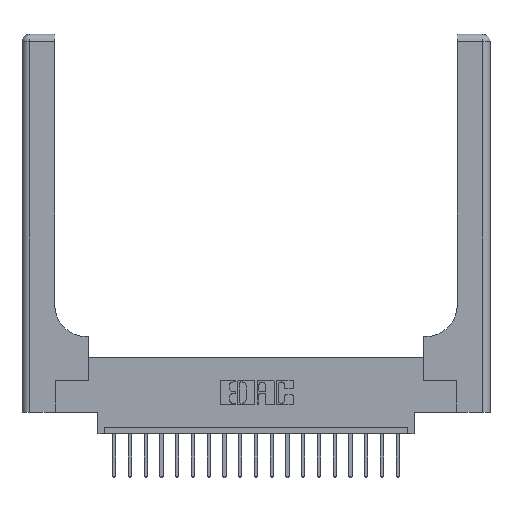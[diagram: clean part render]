
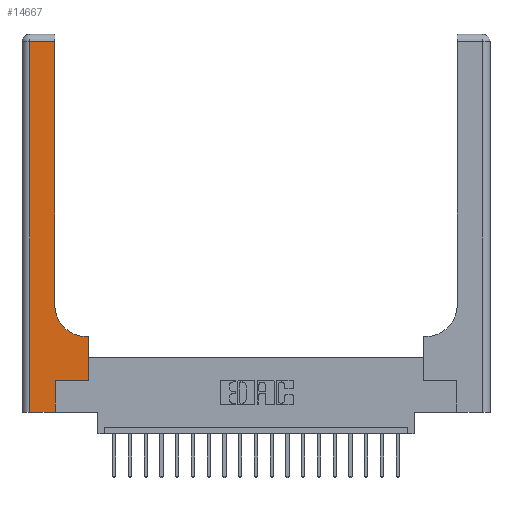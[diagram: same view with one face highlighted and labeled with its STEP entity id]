
A CAD part, top view. The second image highlights one B-rep face of the part: STEP entity #14667.
In plain terms, the highlighted planar face has unit normal (0, 0, 1).
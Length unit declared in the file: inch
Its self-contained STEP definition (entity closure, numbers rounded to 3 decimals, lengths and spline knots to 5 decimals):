
#62 = CARTESIAN_POINT ( 'NONE',  ( 0., 0., 0.37 ) ) ;
#300 = EDGE_CURVE ( 'NONE', #12761, #14336, #6919, .T. ) ;
#1386 = LINE ( 'NONE', #4440, #5822 ) ;
#1417 = DIRECTION ( 'NONE',  ( -1., 0., 0. ) ) ;
#2217 = AXIS2_PLACEMENT_3D ( 'NONE', #19661, #11805, #13181 ) ;
#2531 = ORIENTED_EDGE ( 'NONE', *, *, #5670, .T. ) ;
#2569 = CARTESIAN_POINT ( 'NONE',  ( 0.26, 0.85, 0.37 ) ) ;
#2902 = EDGE_LOOP ( 'NONE', ( #2531, #15123, #10758, #13606, #8999, #5307, #18070, #15414, #9375 ) ) ;
#3786 = CARTESIAN_POINT ( 'NONE',  ( 0.51, 0.6, 0.37 ) ) ;
#4196 = LINE ( 'NONE', #17015, #17598 ) ;
#4314 = FACE_OUTER_BOUND ( 'NONE', #2902, .T. ) ;
#4440 = CARTESIAN_POINT ( 'NONE',  ( 0.06, 3., 0.37 ) ) ;
#4632 = DIRECTION ( 'NONE',  ( 1., 0., 0. ) ) ;
#5137 = VECTOR ( 'NONE', #8084, 39.37008 ) ;
#5307 = ORIENTED_EDGE ( 'NONE', *, *, #8189, .T. ) ;
#5670 = EDGE_CURVE ( 'NONE', #12467, #8063, #4196, .T. ) ;
#5822 = VECTOR ( 'NONE', #18939, 39.37008 ) ;
#5879 = PLANE ( 'NONE',  #17621 ) ;
#6220 = CARTESIAN_POINT ( 'NONE',  ( 0.528, 0.6, 0.37 ) ) ;
#6449 = DIRECTION ( 'NONE',  ( 1., 0., 0. ) ) ;
#6518 = EDGE_CURVE ( 'NONE', #14166, #10309, #1386, .T. ) ;
#6613 = DIRECTION ( 'NONE',  ( 0., 1., 0. ) ) ;
#6919 = LINE ( 'NONE', #7130, #20415 ) ;
#7130 = CARTESIAN_POINT ( 'NONE',  ( 0.528, 0.25, 0.37 ) ) ;
#7758 = CARTESIAN_POINT ( 'NONE',  ( 0., 3., 0.37 ) ) ;
#8004 = CARTESIAN_POINT ( 'NONE',  ( 0.06, 2.94, 0.37 ) ) ;
#8063 = VERTEX_POINT ( 'NONE', #15056 ) ;
#8084 = DIRECTION ( 'NONE',  ( -1., 0., 0. ) ) ;
#8189 = EDGE_CURVE ( 'NONE', #10855, #12761, #18812, .T. ) ;
#8978 = EDGE_CURVE ( 'NONE', #8063, #14166, #17585, .T. ) ;
#8999 = ORIENTED_EDGE ( 'NONE', *, *, #14540, .T. ) ;
#9375 = ORIENTED_EDGE ( 'NONE', *, *, #13316, .T. ) ;
#9525 = CARTESIAN_POINT ( 'NONE',  ( 0.265, 0., 0.37 ) ) ;
#9725 = CARTESIAN_POINT ( 'NONE',  ( 0.265, 0., 0.37 ) ) ;
#10309 = VERTEX_POINT ( 'NONE', #16529 ) ;
#10693 = CARTESIAN_POINT ( 'NONE',  ( 0.528, 0.25, 0.37 ) ) ;
#10758 = ORIENTED_EDGE ( 'NONE', *, *, #6518, .T. ) ;
#10774 = VERTEX_POINT ( 'NONE', #3786 ) ;
#10850 = DIRECTION ( 'NONE',  ( 0., 1., 0. ) ) ;
#10855 = VERTEX_POINT ( 'NONE', #18589 ) ;
#11805 = DIRECTION ( 'NONE',  ( 0., 0., -1. ) ) ;
#12467 = VERTEX_POINT ( 'NONE', #2569 ) ;
#12761 = VERTEX_POINT ( 'NONE', #10693 ) ;
#12777 = LINE ( 'NONE', #9525, #17283 ) ;
#12910 = CIRCLE ( 'NONE', #2217, 0.25 ) ;
#13181 = DIRECTION ( 'NONE',  ( 1., 0., 0. ) ) ;
#13196 = VERTEX_POINT ( 'NONE', #9725 ) ;
#13316 = EDGE_CURVE ( 'NONE', #10774, #12467, #12910, .T. ) ;
#13606 = ORIENTED_EDGE ( 'NONE', *, *, #14167, .T. ) ;
#13852 = LINE ( 'NONE', #13958, #20030 ) ;
#13958 = CARTESIAN_POINT ( 'NONE',  ( 0.26, 0.6, 0.37 ) ) ;
#14007 = DIRECTION ( 'NONE',  ( 0., 0., -1. ) ) ;
#14166 = VERTEX_POINT ( 'NONE', #8004 ) ;
#14167 = EDGE_CURVE ( 'NONE', #10309, #13196, #14371, .T. ) ;
#14336 = VERTEX_POINT ( 'NONE', #6220 ) ;
#14371 = LINE ( 'NONE', #62, #20621 ) ;
#14540 = EDGE_CURVE ( 'NONE', #13196, #10855, #12777, .T. ) ;
#14667 = ADVANCED_FACE ( 'NONE', ( #4314 ), #5879, .F. ) ;
#15056 = CARTESIAN_POINT ( 'NONE',  ( 0.26, 2.94, 0.37 ) ) ;
#15123 = ORIENTED_EDGE ( 'NONE', *, *, #8978, .T. ) ;
#15414 = ORIENTED_EDGE ( 'NONE', *, *, #18834, .T. ) ;
#15670 = CARTESIAN_POINT ( 'NONE',  ( 0.265, 0.25, 0.37 ) ) ;
#16018 = CARTESIAN_POINT ( 'NONE',  ( 0., 2.94, 0.37 ) ) ;
#16529 = CARTESIAN_POINT ( 'NONE',  ( 0.06, 0., 0.37 ) ) ;
#17015 = CARTESIAN_POINT ( 'NONE',  ( 0.26, 3., 0.37 ) ) ;
#17283 = VECTOR ( 'NONE', #6613, 39.37008 ) ;
#17585 = LINE ( 'NONE', #16018, #5137 ) ;
#17598 = VECTOR ( 'NONE', #10850, 39.37008 ) ;
#17621 = AXIS2_PLACEMENT_3D ( 'NONE', #7758, #14007, #20079 ) ;
#17719 = VECTOR ( 'NONE', #4632, 39.37008 ) ;
#17972 = DIRECTION ( 'NONE',  ( 0., 1., 0. ) ) ;
#18070 = ORIENTED_EDGE ( 'NONE', *, *, #300, .T. ) ;
#18589 = CARTESIAN_POINT ( 'NONE',  ( 0.265, 0.25, 0.37 ) ) ;
#18812 = LINE ( 'NONE', #15670, #17719 ) ;
#18834 = EDGE_CURVE ( 'NONE', #14336, #10774, #13852, .T. ) ;
#18939 = DIRECTION ( 'NONE',  ( 0., -1., 0. ) ) ;
#19661 = CARTESIAN_POINT ( 'NONE',  ( 0.51, 0.85, 0.37 ) ) ;
#20030 = VECTOR ( 'NONE', #1417, 39.37008 ) ;
#20079 = DIRECTION ( 'NONE',  ( -1., 0., 0. ) ) ;
#20415 = VECTOR ( 'NONE', #17972, 39.37008 ) ;
#20621 = VECTOR ( 'NONE', #6449, 39.37008 ) ;
